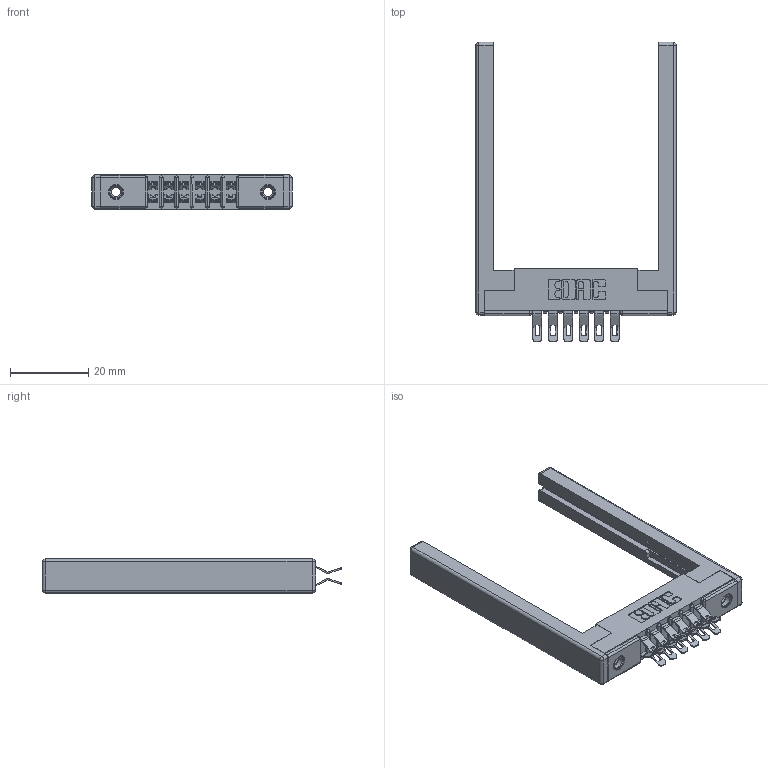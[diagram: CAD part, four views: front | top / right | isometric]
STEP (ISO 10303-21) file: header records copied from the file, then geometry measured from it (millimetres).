
FILE_DESCRIPTION (( 'STEP AP203' ), '1' );
FILE_NAME ('307-012-455-268.STEP', '2020-09-28T14:50:29', ( '' ), ( '' ), 'SwSTEP 2.0', 'SolidWorks 2020', '' );
FILE_SCHEMA (( 'CONFIG_CONTROL_DESIGN' ));
Length unit declared in the file: inch
Products named in the file (5): 307-220-068; 345-250-001_345-250-001-102; 307-290-001_555; 307 Part_.156 Dia Mounting Holes; 307-012-455-268
Assembly tree (17 placements, depth 2):
  307-012-455-268
    307 Part_.156 Dia Mounting Holes
    307-290-001_555  x12
    307-220-068  x2
    345-250-001_345-250-001-102  x2
Bounding box: 51.21 x 76.71 x 8.71 mm (x, y, z)
Volume: 7948.5 mm3; surface area: 9389.3 mm2
Topology: 17 solids, 17 shells, 1011 faces, 2885 edges, 1866 vertices
Faces by surface type: plane 566, cylinder 407, sphere 22, cone 12, torus 4
Entity records: 13070 total; most frequent: CARTESIAN_POINT 2131, DIRECTION 2125, ORIENTED_EDGE 2102, EDGE_CURVE 1051, LINE 777, VECTOR 777, VERTEX_POINT 680, AXIS2_PLACEMENT_3D 674
